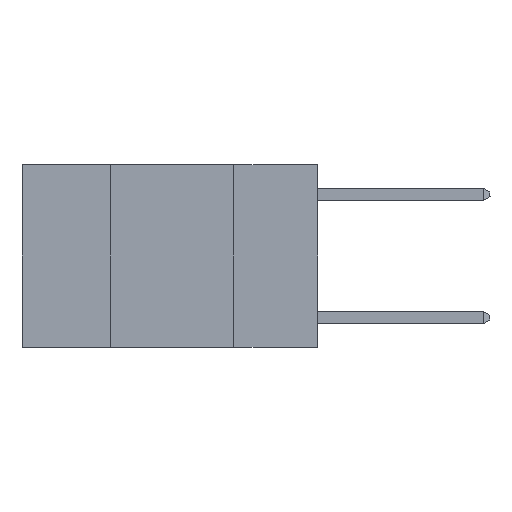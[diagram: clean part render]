
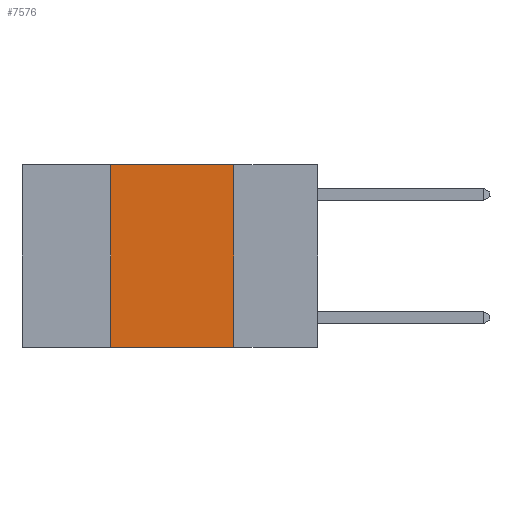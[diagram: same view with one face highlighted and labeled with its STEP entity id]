
A CAD part, left-side view. The second image highlights one B-rep face of the part: STEP entity #7576.
In plain terms, the highlighted planar face has unit normal (-1, 0, 0).
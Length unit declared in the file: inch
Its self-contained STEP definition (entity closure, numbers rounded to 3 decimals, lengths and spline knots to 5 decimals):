
#112 = ORIENTED_EDGE ( 'NONE', *, *, #9577, .T. ) ;
#1144 = CARTESIAN_POINT ( 'NONE',  ( 0., 0.6, 0. ) ) ;
#2010 = LINE ( 'NONE', #25404, #15135 ) ;
#4179 = CARTESIAN_POINT ( 'NONE',  ( 0., 0.17, 0. ) ) ;
#4497 = CARTESIAN_POINT ( 'NONE',  ( 0., 0.17, 0. ) ) ;
#5948 = FACE_OUTER_BOUND ( 'NONE', #26263, .T. ) ;
#6053 = VERTEX_POINT ( 'NONE', #4497 ) ;
#6069 = CARTESIAN_POINT ( 'NONE',  ( 0., 0.6, -0.37 ) ) ;
#6527 = DIRECTION ( 'NONE',  ( 0., -1., 0. ) ) ;
#7576 = ADVANCED_FACE ( 'NONE', ( #5948 ), #29803, .F. ) ;
#8488 = DIRECTION ( 'NONE',  ( 0., -1., 0. ) ) ;
#9577 = EDGE_CURVE ( 'NONE', #21616, #24955, #25268, .T. ) ;
#9893 = ORIENTED_EDGE ( 'NONE', *, *, #23145, .F. ) ;
#11497 = EDGE_CURVE ( 'NONE', #6053, #24955, #20126, .T. ) ;
#13161 = DIRECTION ( 'NONE',  ( 0., 0., 1. ) ) ;
#13505 = VERTEX_POINT ( 'NONE', #22923 ) ;
#13607 = DIRECTION ( 'NONE',  ( 0., 0., -1. ) ) ;
#14086 = VECTOR ( 'NONE', #6527, 39.37008 ) ;
#14926 = DIRECTION ( 'NONE',  ( 0., 0., -1. ) ) ;
#15135 = VECTOR ( 'NONE', #13161, 39.37008 ) ;
#17251 = DIRECTION ( 'NONE',  ( 1., 0., 0. ) ) ;
#19350 = ORIENTED_EDGE ( 'NONE', *, *, #19816, .F. ) ;
#19816 = EDGE_CURVE ( 'NONE', #13505, #6053, #29884, .T. ) ;
#20084 = CARTESIAN_POINT ( 'NONE',  ( 0., 0.42, -0.37 ) ) ;
#20126 = LINE ( 'NONE', #4179, #22102 ) ;
#20562 = CARTESIAN_POINT ( 'NONE',  ( 0., 0.17, -0.37 ) ) ;
#20875 = CARTESIAN_POINT ( 'NONE',  ( 0., 0.6, 0. ) ) ;
#21616 = VERTEX_POINT ( 'NONE', #20084 ) ;
#22102 = VECTOR ( 'NONE', #13607, 39.37008 ) ;
#22923 = CARTESIAN_POINT ( 'NONE',  ( 0., 0.42, 0. ) ) ;
#23145 = EDGE_CURVE ( 'NONE', #21616, #13505, #2010, .T. ) ;
#24955 = VERTEX_POINT ( 'NONE', #20562 ) ;
#25268 = LINE ( 'NONE', #6069, #14086 ) ;
#25404 = CARTESIAN_POINT ( 'NONE',  ( 0., 0.42, 0. ) ) ;
#26263 = EDGE_LOOP ( 'NONE', ( #28132, #19350, #9893, #112 ) ) ;
#26882 = AXIS2_PLACEMENT_3D ( 'NONE', #1144, #17251, #14926 ) ;
#27826 = VECTOR ( 'NONE', #8488, 39.37008 ) ;
#28132 = ORIENTED_EDGE ( 'NONE', *, *, #11497, .F. ) ;
#29803 = PLANE ( 'NONE',  #26882 ) ;
#29884 = LINE ( 'NONE', #20875, #27826 ) ;
